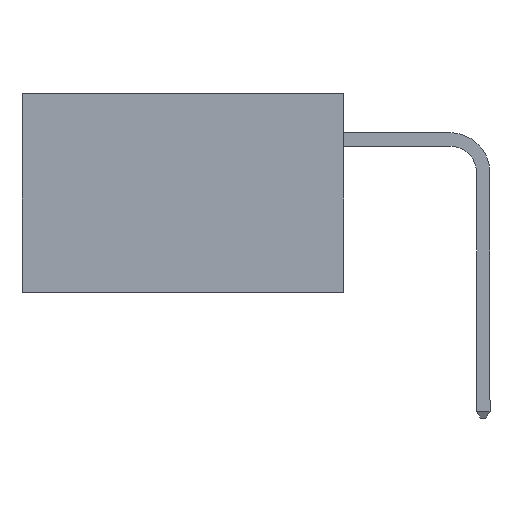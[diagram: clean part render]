
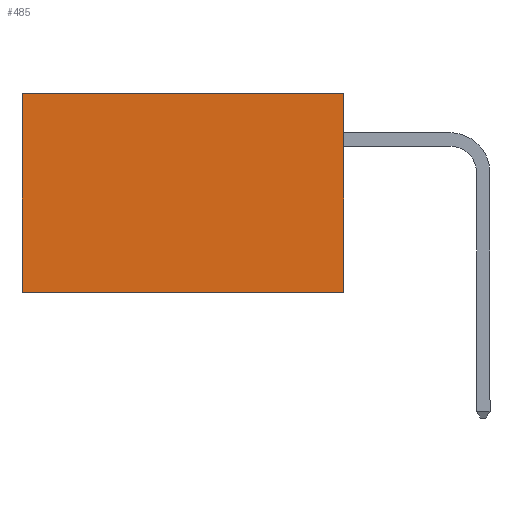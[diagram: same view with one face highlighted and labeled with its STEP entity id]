
A CAD part, left-side view. The second image highlights one B-rep face of the part: STEP entity #485.
In plain terms, the highlighted planar face has unit normal (-1, 0, 0).
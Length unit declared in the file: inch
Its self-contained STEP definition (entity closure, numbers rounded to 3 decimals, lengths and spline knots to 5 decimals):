
#111 = CARTESIAN_POINT ( 'NONE',  ( 0.2615, 0.6, -0.37 ) ) ;
#175 = VECTOR ( 'NONE', #7066, 39.37008 ) ;
#416 = VERTEX_POINT ( 'NONE', #564 ) ;
#438 = LINE ( 'NONE', #3742, #2082 ) ;
#485 = ADVANCED_FACE ( 'NONE', ( #876 ), #9505, .F. ) ;
#564 = CARTESIAN_POINT ( 'NONE',  ( 0.2615, 0., 0. ) ) ;
#632 = VERTEX_POINT ( 'NONE', #7743 ) ;
#876 = FACE_OUTER_BOUND ( 'NONE', #3018, .T. ) ;
#1116 = EDGE_CURVE ( 'NONE', #7359, #1754, #438, .T. ) ;
#1171 = VECTOR ( 'NONE', #6536, 39.37008 ) ;
#1754 = VERTEX_POINT ( 'NONE', #111 ) ;
#2010 = VECTOR ( 'NONE', #5485, 39.37008 ) ;
#2082 = VECTOR ( 'NONE', #3645, 39.37008 ) ;
#2702 = CARTESIAN_POINT ( 'NONE',  ( 0.2615, 0.6, 0. ) ) ;
#3018 = EDGE_LOOP ( 'NONE', ( #3596, #3657, #3668, #3717 ) ) ;
#3389 = CARTESIAN_POINT ( 'NONE',  ( 0.2615, 0., -0.37 ) ) ;
#3596 = ORIENTED_EDGE ( 'NONE', *, *, #1116, .T. ) ;
#3645 = DIRECTION ( 'NONE',  ( 0., 0., -1. ) ) ;
#3657 = ORIENTED_EDGE ( 'NONE', *, *, #6999, .F. ) ;
#3668 = ORIENTED_EDGE ( 'NONE', *, *, #9518, .F. ) ;
#3717 = ORIENTED_EDGE ( 'NONE', *, *, #6876, .T. ) ;
#3742 = CARTESIAN_POINT ( 'NONE',  ( 0.2615, 0.6, -0.37 ) ) ;
#5404 = CARTESIAN_POINT ( 'NONE',  ( 0.2615, 0., -0.37 ) ) ;
#5485 = DIRECTION ( 'NONE',  ( 0., 1., 0. ) ) ;
#6230 = LINE ( 'NONE', #5404, #2010 ) ;
#6536 = DIRECTION ( 'NONE',  ( 0., 1., 0. ) ) ;
#6607 = CARTESIAN_POINT ( 'NONE',  ( 0.2615, 0., 0. ) ) ;
#6876 = EDGE_CURVE ( 'NONE', #416, #7359, #8969, .T. ) ;
#6999 = EDGE_CURVE ( 'NONE', #632, #1754, #6230, .T. ) ;
#7066 = DIRECTION ( 'NONE',  ( 0., 0., -1. ) ) ;
#7359 = VERTEX_POINT ( 'NONE', #2702 ) ;
#7743 = CARTESIAN_POINT ( 'NONE',  ( 0.2615, 0., -0.37 ) ) ;
#7983 = LINE ( 'NONE', #3389, #175 ) ;
#8361 = AXIS2_PLACEMENT_3D ( 'NONE', #9387, #9370, #9366 ) ;
#8969 = LINE ( 'NONE', #6607, #1171 ) ;
#9366 = DIRECTION ( 'NONE',  ( 0., 0., -1. ) ) ;
#9370 = DIRECTION ( 'NONE',  ( 1., 0., 0. ) ) ;
#9387 = CARTESIAN_POINT ( 'NONE',  ( 0.2615, 0., -0.37 ) ) ;
#9505 = PLANE ( 'NONE',  #8361 ) ;
#9518 = EDGE_CURVE ( 'NONE', #416, #632, #7983, .T. ) ;
